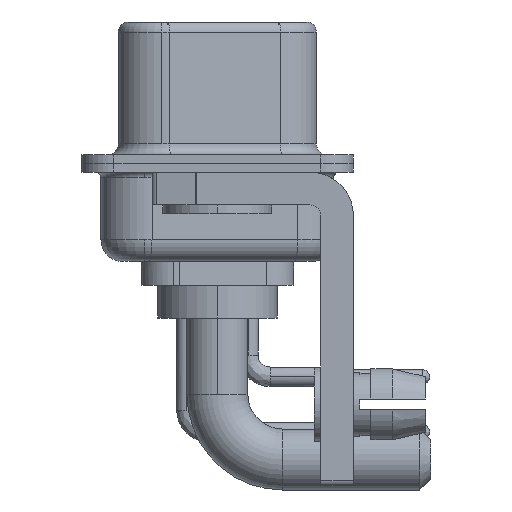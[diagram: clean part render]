
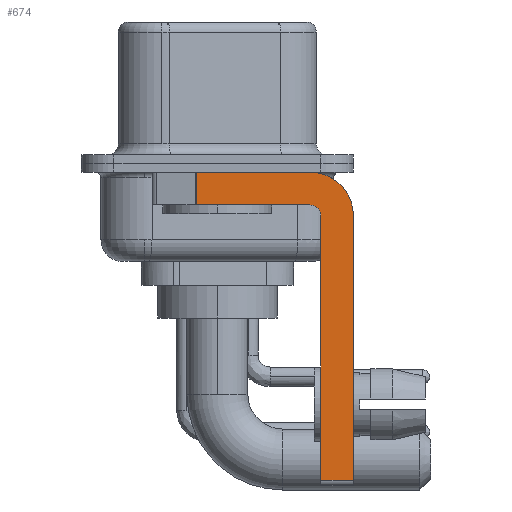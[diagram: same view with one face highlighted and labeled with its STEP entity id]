
A CAD part, left-side view. The second image highlights one B-rep face of the part: STEP entity #674.
In plain terms, the highlighted planar face has unit normal (-1, 0, 0).
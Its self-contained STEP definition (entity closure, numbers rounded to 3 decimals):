
#218 = VERTEX_POINT ( 'NONE', #11683 ) ;
#567 = VECTOR ( 'NONE', #23248, 1000. ) ;
#674 = ADVANCED_FACE ( 'NONE', ( #13684 ), #18843, .F. ) ;
#712 = EDGE_CURVE ( 'NONE', #20029, #10327, #2390, .T. ) ;
#794 = CARTESIAN_POINT ( 'NONE',  ( -2.9, -4.75, -14.8 ) ) ;
#813 = EDGE_CURVE ( 'NONE', #29389, #5083, #29419, .T. ) ;
#940 = DIRECTION ( 'NONE',  ( 0., -1., 0. ) ) ;
#1359 = ORIENTED_EDGE ( 'NONE', *, *, #16977, .F. ) ;
#1376 = DIRECTION ( 'NONE',  ( 1., 0., 0. ) ) ;
#2390 = LINE ( 'NONE', #18386, #22226 ) ;
#3316 = ORIENTED_EDGE ( 'NONE', *, *, #8272, .F. ) ;
#4276 = CARTESIAN_POINT ( 'NONE',  ( -2.9, -4.25, -0.4 ) ) ;
#5083 = VERTEX_POINT ( 'NONE', #4276 ) ;
#5095 = EDGE_CURVE ( 'NONE', #218, #9991, #16345, .T. ) ;
#5305 = VECTOR ( 'NONE', #10338, 1000. ) ;
#5307 = DIRECTION ( 'NONE',  ( -1., 0., 0. ) ) ;
#5595 = CARTESIAN_POINT ( 'NONE',  ( -2.9, 0.978, -1.9 ) ) ;
#5949 = AXIS2_PLACEMENT_3D ( 'NONE', #7052, #5307, #14865 ) ;
#6047 = LINE ( 'NONE', #8845, #567 ) ;
#6118 = CARTESIAN_POINT ( 'NONE',  ( -2.9, -4.75, -14.55 ) ) ;
#6482 = DIRECTION ( 'NONE',  ( 0., 0., -1. ) ) ;
#7052 = CARTESIAN_POINT ( 'NONE',  ( -2.9, -4.25, -2.4 ) ) ;
#7629 = ORIENTED_EDGE ( 'NONE', *, *, #16694, .F. ) ;
#8096 = LINE ( 'NONE', #5595, #15647 ) ;
#8272 = EDGE_CURVE ( 'NONE', #20029, #17105, #10514, .T. ) ;
#8460 = CIRCLE ( 'NONE', #9457, 2. ) ;
#8845 = CARTESIAN_POINT ( 'NONE',  ( -2.9, -6.25, -2.4 ) ) ;
#9457 = AXIS2_PLACEMENT_3D ( 'NONE', #30027, #1376, #20641 ) ;
#9991 = VERTEX_POINT ( 'NONE', #15749 ) ;
#10327 = VERTEX_POINT ( 'NONE', #19251 ) ;
#10338 = DIRECTION ( 'NONE',  ( 0., 0., 1. ) ) ;
#10514 = LINE ( 'NONE', #794, #5305 ) ;
#10736 = DIRECTION ( 'NONE',  ( 0., 0., -1. ) ) ;
#11568 = EDGE_LOOP ( 'NONE', ( #23828, #14520, #28062, #7629, #3316, #18380, #22278, #1359 ) ) ;
#11683 = CARTESIAN_POINT ( 'NONE',  ( -2.9, -4.25, -1.9 ) ) ;
#13684 = FACE_OUTER_BOUND ( 'NONE', #11568, .T. ) ;
#13691 = CARTESIAN_POINT ( 'NONE',  ( -2.9, -4.25, -1.9 ) ) ;
#14102 = CARTESIAN_POINT ( 'NONE',  ( -2.9, -6.25, -2.4 ) ) ;
#14108 = EDGE_CURVE ( 'NONE', #15197, #10327, #6047, .T. ) ;
#14520 = ORIENTED_EDGE ( 'NONE', *, *, #21072, .T. ) ;
#14865 = DIRECTION ( 'NONE',  ( 0., 0., 1. ) ) ;
#15197 = VERTEX_POINT ( 'NONE', #14102 ) ;
#15647 = VECTOR ( 'NONE', #10736, 1000. ) ;
#15749 = CARTESIAN_POINT ( 'NONE',  ( -2.9, 0.978, -1.9 ) ) ;
#16345 = LINE ( 'NONE', #13691, #25517 ) ;
#16694 = EDGE_CURVE ( 'NONE', #17105, #218, #19470, .T. ) ;
#16977 = EDGE_CURVE ( 'NONE', #5083, #15197, #8460, .T. ) ;
#17105 = VERTEX_POINT ( 'NONE', #21575 ) ;
#17689 = CARTESIAN_POINT ( 'NONE',  ( -2.9, 3., -0.4 ) ) ;
#18380 = ORIENTED_EDGE ( 'NONE', *, *, #712, .T. ) ;
#18386 = CARTESIAN_POINT ( 'NONE',  ( -2.9, -4.25, -14.55 ) ) ;
#18843 = PLANE ( 'NONE',  #20729 ) ;
#19251 = CARTESIAN_POINT ( 'NONE',  ( -2.9, -6.25, -14.55 ) ) ;
#19470 = CIRCLE ( 'NONE', #5949, 0.5 ) ;
#20029 = VERTEX_POINT ( 'NONE', #6118 ) ;
#20641 = DIRECTION ( 'NONE',  ( 0., 0., -1. ) ) ;
#20729 = AXIS2_PLACEMENT_3D ( 'NONE', #27906, #23837, #6482 ) ;
#21072 = EDGE_CURVE ( 'NONE', #29389, #9991, #8096, .T. ) ;
#21575 = CARTESIAN_POINT ( 'NONE',  ( -2.9, -4.75, -2.4 ) ) ;
#22226 = VECTOR ( 'NONE', #30708, 1000. ) ;
#22278 = ORIENTED_EDGE ( 'NONE', *, *, #14108, .F. ) ;
#22748 = VECTOR ( 'NONE', #940, 1000. ) ;
#23248 = DIRECTION ( 'NONE',  ( 0., 0., -1. ) ) ;
#23828 = ORIENTED_EDGE ( 'NONE', *, *, #813, .F. ) ;
#23837 = DIRECTION ( 'NONE',  ( 1., 0., 0. ) ) ;
#25517 = VECTOR ( 'NONE', #25884, 1000. ) ;
#25884 = DIRECTION ( 'NONE',  ( 0., 1., 0. ) ) ;
#26379 = CARTESIAN_POINT ( 'NONE',  ( -2.9, 0.978, -0.4 ) ) ;
#27906 = CARTESIAN_POINT ( 'NONE',  ( -2.9, -4.25, -2.4 ) ) ;
#28062 = ORIENTED_EDGE ( 'NONE', *, *, #5095, .F. ) ;
#29389 = VERTEX_POINT ( 'NONE', #26379 ) ;
#29419 = LINE ( 'NONE', #17689, #22748 ) ;
#30027 = CARTESIAN_POINT ( 'NONE',  ( -2.9, -4.25, -2.4 ) ) ;
#30708 = DIRECTION ( 'NONE',  ( 0., -1., 0. ) ) ;
